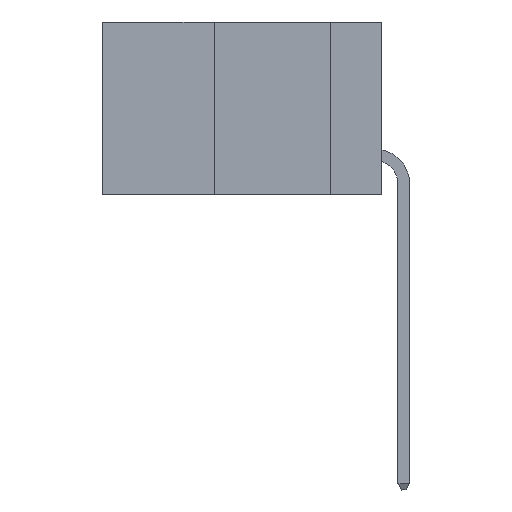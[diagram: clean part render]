
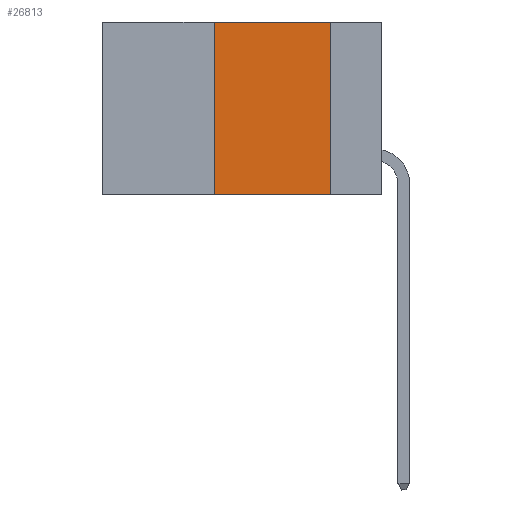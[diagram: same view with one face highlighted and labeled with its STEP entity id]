
A CAD part, left-side view. The second image highlights one B-rep face of the part: STEP entity #26813.
In plain terms, the highlighted planar face has unit normal (-1, 0, 0).
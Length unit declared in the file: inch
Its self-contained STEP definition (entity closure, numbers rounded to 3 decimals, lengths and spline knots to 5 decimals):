
#723 = EDGE_LOOP ( 'NONE', ( #10056, #18994, #4639, #12331 ) ) ;
#2011 = VECTOR ( 'NONE', #12764, 39.37008 ) ;
#2534 = VECTOR ( 'NONE', #6625, 39.37008 ) ;
#2612 = AXIS2_PLACEMENT_3D ( 'NONE', #10714, #6407, #17082 ) ;
#2820 = CARTESIAN_POINT ( 'NONE',  ( 0., 0.6, 0. ) ) ;
#2900 = LINE ( 'NONE', #19719, #2534 ) ;
#3693 = VERTEX_POINT ( 'NONE', #13912 ) ;
#4639 = ORIENTED_EDGE ( 'NONE', *, *, #10843, .F. ) ;
#6090 = CARTESIAN_POINT ( 'NONE',  ( 0., 0.36, 0. ) ) ;
#6360 = CARTESIAN_POINT ( 'NONE',  ( 0., 0.6, -0.37 ) ) ;
#6407 = DIRECTION ( 'NONE',  ( 1., 0., 0. ) ) ;
#6625 = DIRECTION ( 'NONE',  ( 0., 0., -1. ) ) ;
#7718 = LINE ( 'NONE', #2820, #2011 ) ;
#8182 = FACE_OUTER_BOUND ( 'NONE', #723, .T. ) ;
#8480 = PLANE ( 'NONE',  #2612 ) ;
#10056 = ORIENTED_EDGE ( 'NONE', *, *, #25030, .F. ) ;
#10714 = CARTESIAN_POINT ( 'NONE',  ( 0., 0.6, 0. ) ) ;
#10843 = EDGE_CURVE ( 'NONE', #21742, #24629, #18327, .T. ) ;
#11369 = VECTOR ( 'NONE', #20949, 39.37008 ) ;
#12331 = ORIENTED_EDGE ( 'NONE', *, *, #24890, .T. ) ;
#12468 = EDGE_CURVE ( 'NONE', #24629, #18922, #7718, .T. ) ;
#12764 = DIRECTION ( 'NONE',  ( 0., -1., 0. ) ) ;
#13233 = LINE ( 'NONE', #6360, #15198 ) ;
#13912 = CARTESIAN_POINT ( 'NONE',  ( 0., 0.11, -0.37 ) ) ;
#14430 = CARTESIAN_POINT ( 'NONE',  ( 0., 0.11, 0. ) ) ;
#15198 = VECTOR ( 'NONE', #21222, 39.37008 ) ;
#17082 = DIRECTION ( 'NONE',  ( 0., 0., -1. ) ) ;
#17840 = CARTESIAN_POINT ( 'NONE',  ( 0., 0.36, -0.37 ) ) ;
#18327 = LINE ( 'NONE', #6090, #11369 ) ;
#18922 = VERTEX_POINT ( 'NONE', #14430 ) ;
#18994 = ORIENTED_EDGE ( 'NONE', *, *, #12468, .F. ) ;
#19719 = CARTESIAN_POINT ( 'NONE',  ( 0., 0.11, 0. ) ) ;
#20949 = DIRECTION ( 'NONE',  ( 0., 0., 1. ) ) ;
#21222 = DIRECTION ( 'NONE',  ( 0., -1., 0. ) ) ;
#21742 = VERTEX_POINT ( 'NONE', #17840 ) ;
#23316 = CARTESIAN_POINT ( 'NONE',  ( 0., 0.36, 0. ) ) ;
#24629 = VERTEX_POINT ( 'NONE', #23316 ) ;
#24890 = EDGE_CURVE ( 'NONE', #21742, #3693, #13233, .T. ) ;
#25030 = EDGE_CURVE ( 'NONE', #18922, #3693, #2900, .T. ) ;
#26813 = ADVANCED_FACE ( 'NONE', ( #8182 ), #8480, .F. ) ;
